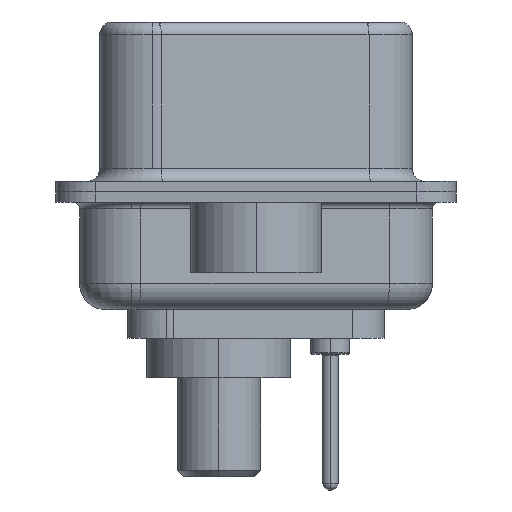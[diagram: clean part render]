
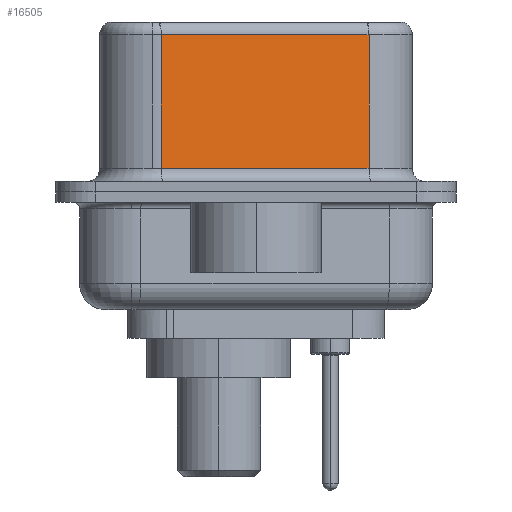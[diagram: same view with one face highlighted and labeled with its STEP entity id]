
A CAD part, left-side view. The second image highlights one B-rep face of the part: STEP entity #16505.
In plain terms, the highlighted planar face has unit normal (-0.985, -0.174, 0).
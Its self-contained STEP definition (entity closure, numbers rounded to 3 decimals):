
#116 = VERTEX_POINT ( 'NONE', #21150 ) ;
#1043 = FACE_OUTER_BOUND ( 'NONE', #18741, .T. ) ;
#1045 = CARTESIAN_POINT ( 'NONE',  ( 5.132, -4.322, 0.9 ) ) ;
#1622 = ORIENTED_EDGE ( 'NONE', *, *, #20868, .T. ) ;
#1700 = PLANE ( 'NONE',  #18563 ) ;
#2371 = VECTOR ( 'NONE', #5156, 1000. ) ;
#2705 = DIRECTION ( 'NONE',  ( 0.174, -0.985, 0. ) ) ;
#3573 = CARTESIAN_POINT ( 'NONE',  ( 3.73, 3.628, 6.52 ) ) ;
#5065 = DIRECTION ( 'NONE',  ( 0., 0., -1. ) ) ;
#5156 = DIRECTION ( 'NONE',  ( 0., 0., -1. ) ) ;
#5537 = LINE ( 'NONE', #3573, #15212 ) ;
#6630 = DIRECTION ( 'NONE',  ( -0.174, 0.985, 0. ) ) ;
#7186 = CARTESIAN_POINT ( 'NONE',  ( 5.132, -4.322, 0.9 ) ) ;
#7859 = VECTOR ( 'NONE', #20859, 1000. ) ;
#8169 = CARTESIAN_POINT ( 'NONE',  ( 5.132, -4.322, 6.52 ) ) ;
#9053 = CARTESIAN_POINT ( 'NONE',  ( 3.73, 3.628, 0.9 ) ) ;
#9389 = VERTEX_POINT ( 'NONE', #9053 ) ;
#9538 = EDGE_CURVE ( 'NONE', #13113, #116, #12202, .T. ) ;
#9867 = VERTEX_POINT ( 'NONE', #7186 ) ;
#10422 = LINE ( 'NONE', #1045, #18630 ) ;
#11527 = CARTESIAN_POINT ( 'NONE',  ( 5.132, -4.322, 6.52 ) ) ;
#12049 = LINE ( 'NONE', #11527, #2371 ) ;
#12202 = LINE ( 'NONE', #19184, #7859 ) ;
#13113 = VERTEX_POINT ( 'NONE', #16831 ) ;
#13898 = ORIENTED_EDGE ( 'NONE', *, *, #16118, .F. ) ;
#14582 = ORIENTED_EDGE ( 'NONE', *, *, #9538, .T. ) ;
#15212 = VECTOR ( 'NONE', #5065, 1000. ) ;
#16118 = EDGE_CURVE ( 'NONE', #13113, #9867, #12049, .T. ) ;
#16399 = DIRECTION ( 'NONE',  ( 0.985, 0.174, 0. ) ) ;
#16505 = ADVANCED_FACE ( 'NONE', ( #1043 ), #1700, .F. ) ;
#16831 = CARTESIAN_POINT ( 'NONE',  ( 5.132, -4.322, 6.02 ) ) ;
#18563 = AXIS2_PLACEMENT_3D ( 'NONE', #8169, #16399, #6630 ) ;
#18630 = VECTOR ( 'NONE', #2705, 1000. ) ;
#18741 = EDGE_LOOP ( 'NONE', ( #13898, #14582, #1622, #20262 ) ) ;
#18750 = EDGE_CURVE ( 'NONE', #9389, #9867, #10422, .T. ) ;
#19184 = CARTESIAN_POINT ( 'NONE',  ( 5.132, -4.322, 6.02 ) ) ;
#20262 = ORIENTED_EDGE ( 'NONE', *, *, #18750, .T. ) ;
#20859 = DIRECTION ( 'NONE',  ( -0.174, 0.985, 0. ) ) ;
#20868 = EDGE_CURVE ( 'NONE', #116, #9389, #5537, .T. ) ;
#21150 = CARTESIAN_POINT ( 'NONE',  ( 3.73, 3.628, 6.02 ) ) ;
